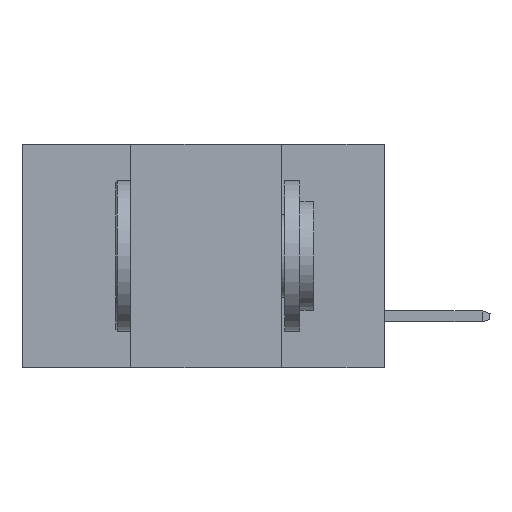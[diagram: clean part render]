
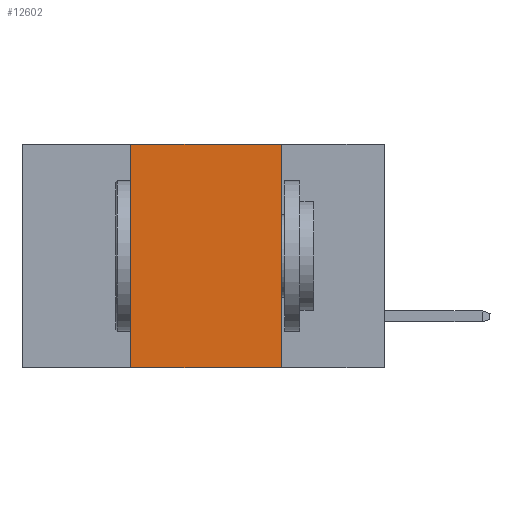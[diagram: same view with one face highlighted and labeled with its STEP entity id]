
A CAD part, left-side view. The second image highlights one B-rep face of the part: STEP entity #12602.
In plain terms, the highlighted planar face has unit normal (-1, 0, 0).
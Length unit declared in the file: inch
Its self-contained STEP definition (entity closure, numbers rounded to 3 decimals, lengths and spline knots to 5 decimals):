
#879 = LINE ( 'NONE', #13475, #911 ) ;
#911 = VECTOR ( 'NONE', #10759, 39.37008 ) ;
#1181 = CARTESIAN_POINT ( 'NONE',  ( 0., 0.6, 0. ) ) ;
#2452 = ORIENTED_EDGE ( 'NONE', *, *, #13269, .T. ) ;
#2536 = LINE ( 'NONE', #12258, #3917 ) ;
#3403 = CARTESIAN_POINT ( 'NONE',  ( 0., 0.42, -0.37 ) ) ;
#3801 = DIRECTION ( 'NONE',  ( 0., -1., 0. ) ) ;
#3917 = VECTOR ( 'NONE', #6867, 39.37008 ) ;
#4601 = CARTESIAN_POINT ( 'NONE',  ( 0., 0.17, 0. ) ) ;
#4761 = EDGE_CURVE ( 'NONE', #11020, #7578, #879, .T. ) ;
#4817 = CARTESIAN_POINT ( 'NONE',  ( 0., 0.6, -0.37 ) ) ;
#4933 = CARTESIAN_POINT ( 'NONE',  ( 0., 0.42, 0. ) ) ;
#5454 = DIRECTION ( 'NONE',  ( 0., -1., 0. ) ) ;
#5683 = EDGE_LOOP ( 'NONE', ( #13132, #10172, #9733, #2452 ) ) ;
#6056 = VERTEX_POINT ( 'NONE', #7097 ) ;
#6125 = DIRECTION ( 'NONE',  ( 0., 0., -1. ) ) ;
#6867 = DIRECTION ( 'NONE',  ( 0., 0., -1. ) ) ;
#7088 = VECTOR ( 'NONE', #3801, 39.37008 ) ;
#7097 = CARTESIAN_POINT ( 'NONE',  ( 0., 0.17, -0.37 ) ) ;
#7459 = DIRECTION ( 'NONE',  ( 1., 0., 0. ) ) ;
#7578 = VERTEX_POINT ( 'NONE', #4933 ) ;
#8833 = EDGE_CURVE ( 'NONE', #7578, #13180, #9699, .T. ) ;
#9699 = LINE ( 'NONE', #1181, #10428 ) ;
#9733 = ORIENTED_EDGE ( 'NONE', *, *, #4761, .F. ) ;
#10172 = ORIENTED_EDGE ( 'NONE', *, *, #8833, .F. ) ;
#10428 = VECTOR ( 'NONE', #5454, 39.37008 ) ;
#10649 = FACE_OUTER_BOUND ( 'NONE', #5683, .T. ) ;
#10759 = DIRECTION ( 'NONE',  ( 0., 0., 1. ) ) ;
#10929 = AXIS2_PLACEMENT_3D ( 'NONE', #13906, #7459, #6125 ) ;
#11020 = VERTEX_POINT ( 'NONE', #3403 ) ;
#11256 = LINE ( 'NONE', #4817, #7088 ) ;
#12258 = CARTESIAN_POINT ( 'NONE',  ( 0., 0.17, -0.37 ) ) ;
#12602 = ADVANCED_FACE ( 'NONE', ( #10649 ), #13700, .F. ) ;
#13132 = ORIENTED_EDGE ( 'NONE', *, *, #13241, .F. ) ;
#13180 = VERTEX_POINT ( 'NONE', #4601 ) ;
#13241 = EDGE_CURVE ( 'NONE', #13180, #6056, #2536, .T. ) ;
#13269 = EDGE_CURVE ( 'NONE', #11020, #6056, #11256, .T. ) ;
#13475 = CARTESIAN_POINT ( 'NONE',  ( 0., 0.42, -0.37 ) ) ;
#13700 = PLANE ( 'NONE',  #10929 ) ;
#13906 = CARTESIAN_POINT ( 'NONE',  ( 0., 0.6, 0. ) ) ;
